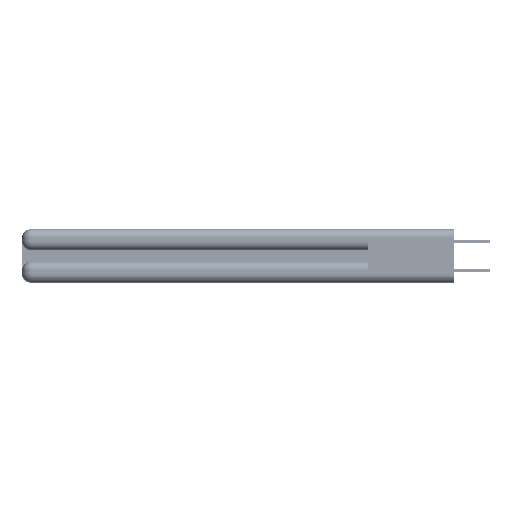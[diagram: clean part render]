
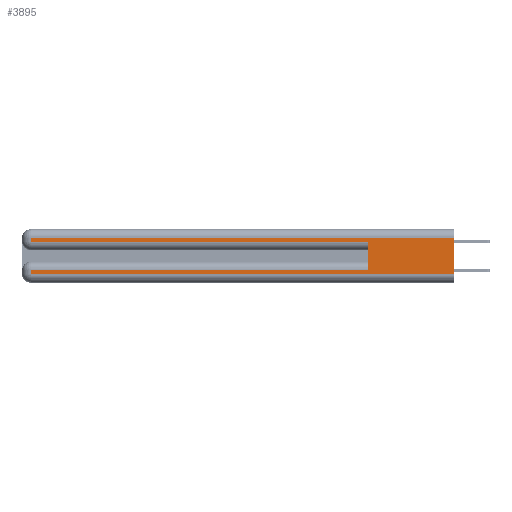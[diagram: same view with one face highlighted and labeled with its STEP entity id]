
A CAD part, left-side view. The second image highlights one B-rep face of the part: STEP entity #3895.
In plain terms, the highlighted planar face has unit normal (-1, 0, 0).
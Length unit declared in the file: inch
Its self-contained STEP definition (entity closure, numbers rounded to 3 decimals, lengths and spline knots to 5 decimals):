
#30 = EDGE_CURVE ( 'NONE', #7439, #9168, #42446, .T. ) ;
#1286 = VERTEX_POINT ( 'NONE', #32134 ) ;
#2136 = LINE ( 'NONE', #8414, #11744 ) ;
#3321 = EDGE_CURVE ( 'NONE', #19346, #48252, #10494, .T. ) ;
#3498 = VECTOR ( 'NONE', #15517, 39.37008 ) ;
#3671 = PLANE ( 'NONE',  #19533 ) ;
#3895 = ADVANCED_FACE ( 'NONE', ( #33763 ), #3671, .F. ) ;
#4121 = CARTESIAN_POINT ( 'NONE',  ( 0., 2.94, 0.085 ) ) ;
#6099 = EDGE_CURVE ( 'NONE', #9168, #19346, #42019, .T. ) ;
#7007 = CARTESIAN_POINT ( 'NONE',  ( 0., 0., 0.37 ) ) ;
#7439 = VERTEX_POINT ( 'NONE', #34771 ) ;
#8203 = VERTEX_POINT ( 'NONE', #32200 ) ;
#8414 = CARTESIAN_POINT ( 'NONE',  ( 0., 0., 0.085 ) ) ;
#9063 = VECTOR ( 'NONE', #38774, 39.37008 ) ;
#9168 = VERTEX_POINT ( 'NONE', #34927 ) ;
#9905 = ORIENTED_EDGE ( 'NONE', *, *, #30, .T. ) ;
#9974 = LINE ( 'NONE', #29205, #25559 ) ;
#10494 = LINE ( 'NONE', #41654, #11077 ) ;
#11077 = VECTOR ( 'NONE', #23205, 39.37008 ) ;
#11744 = VECTOR ( 'NONE', #26841, 39.37008 ) ;
#11901 = VERTEX_POINT ( 'NONE', #45391 ) ;
#12118 = LINE ( 'NONE', #33425, #39063 ) ;
#13740 = VECTOR ( 'NONE', #26459, 39.37008 ) ;
#14959 = EDGE_CURVE ( 'NONE', #1286, #48252, #19552, .T. ) ;
#15215 = EDGE_LOOP ( 'NONE', ( #22426, #9905, #46401, #22282, #35303, #26909, #32712, #41017 ) ) ;
#15265 = DIRECTION ( 'NONE',  ( 1., 0., 0. ) ) ;
#15517 = DIRECTION ( 'NONE',  ( 0., 1., 0. ) ) ;
#17521 = EDGE_CURVE ( 'NONE', #11901, #8203, #9974, .T. ) ;
#18900 = CARTESIAN_POINT ( 'NONE',  ( 0., 0., 0.37 ) ) ;
#19346 = VERTEX_POINT ( 'NONE', #33777 ) ;
#19533 = AXIS2_PLACEMENT_3D ( 'NONE', #18900, #15265, #43168 ) ;
#19552 = LINE ( 'NONE', #41391, #38132 ) ;
#22282 = ORIENTED_EDGE ( 'NONE', *, *, #3321, .T. ) ;
#22426 = ORIENTED_EDGE ( 'NONE', *, *, #31597, .F. ) ;
#23205 = DIRECTION ( 'NONE',  ( 0., -1., 0. ) ) ;
#24776 = EDGE_CURVE ( 'NONE', #45206, #11901, #12118, .T. ) ;
#25559 = VECTOR ( 'NONE', #36258, 39.37008 ) ;
#26459 = DIRECTION ( 'NONE',  ( 0., 0., -1. ) ) ;
#26841 = DIRECTION ( 'NONE',  ( 0., 1., 0. ) ) ;
#26909 = ORIENTED_EDGE ( 'NONE', *, *, #41213, .T. ) ;
#29205 = CARTESIAN_POINT ( 'NONE',  ( 0., 0., 0.06 ) ) ;
#30079 = DIRECTION ( 'NONE',  ( 0., 0., -1. ) ) ;
#31597 = EDGE_CURVE ( 'NONE', #7439, #8203, #34050, .T. ) ;
#32134 = CARTESIAN_POINT ( 'NONE',  ( 0., 0.6, 0.085 ) ) ;
#32200 = CARTESIAN_POINT ( 'NONE',  ( 0., 0., 0.06 ) ) ;
#32712 = ORIENTED_EDGE ( 'NONE', *, *, #24776, .T. ) ;
#33425 = CARTESIAN_POINT ( 'NONE',  ( 0., 2.94, 0.37 ) ) ;
#33763 = FACE_OUTER_BOUND ( 'NONE', #15215, .T. ) ;
#33777 = CARTESIAN_POINT ( 'NONE',  ( 0., 2.94, 0.285 ) ) ;
#33840 = DIRECTION ( 'NONE',  ( 0., 0., 1. ) ) ;
#34050 = LINE ( 'NONE', #7007, #13740 ) ;
#34387 = CARTESIAN_POINT ( 'NONE',  ( 0., 2.94, 0.37 ) ) ;
#34771 = CARTESIAN_POINT ( 'NONE',  ( 0., 0., 0.31 ) ) ;
#34927 = CARTESIAN_POINT ( 'NONE',  ( 0., 2.94, 0.31 ) ) ;
#35303 = ORIENTED_EDGE ( 'NONE', *, *, #14959, .F. ) ;
#36258 = DIRECTION ( 'NONE',  ( 0., -1., 0. ) ) ;
#38132 = VECTOR ( 'NONE', #33840, 39.37008 ) ;
#38774 = DIRECTION ( 'NONE',  ( 0., 0., -1. ) ) ;
#39063 = VECTOR ( 'NONE', #30079, 39.37008 ) ;
#41017 = ORIENTED_EDGE ( 'NONE', *, *, #17521, .T. ) ;
#41213 = EDGE_CURVE ( 'NONE', #1286, #45206, #2136, .T. ) ;
#41391 = CARTESIAN_POINT ( 'NONE',  ( 0., 0.6, 0.145 ) ) ;
#41654 = CARTESIAN_POINT ( 'NONE',  ( 0., 0., 0.285 ) ) ;
#42019 = LINE ( 'NONE', #34387, #9063 ) ;
#42446 = LINE ( 'NONE', #49751, #3498 ) ;
#43168 = DIRECTION ( 'NONE',  ( 0., 0., -1. ) ) ;
#45206 = VERTEX_POINT ( 'NONE', #4121 ) ;
#45391 = CARTESIAN_POINT ( 'NONE',  ( 0., 2.94, 0.06 ) ) ;
#46401 = ORIENTED_EDGE ( 'NONE', *, *, #6099, .T. ) ;
#48252 = VERTEX_POINT ( 'NONE', #49573 ) ;
#49573 = CARTESIAN_POINT ( 'NONE',  ( 0., 0.6, 0.285 ) ) ;
#49751 = CARTESIAN_POINT ( 'NONE',  ( 0., 0., 0.31 ) ) ;
